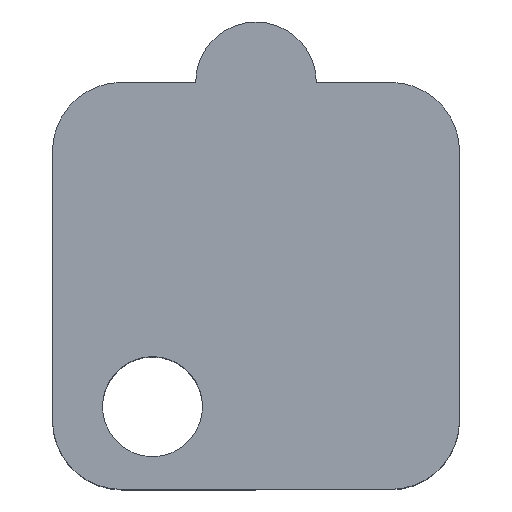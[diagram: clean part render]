
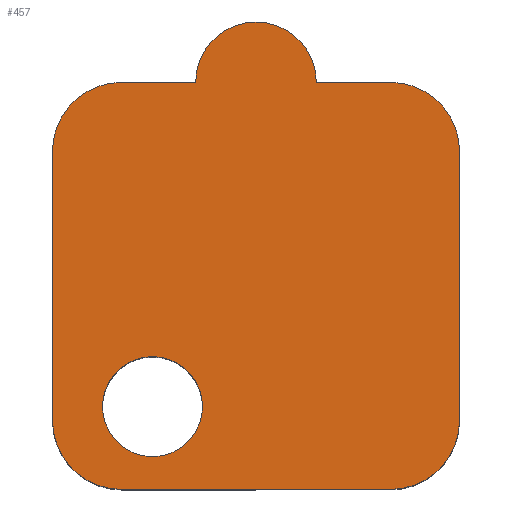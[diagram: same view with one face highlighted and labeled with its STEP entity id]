
A CAD part, top view. The second image highlights one B-rep face of the part: STEP entity #457.
In plain terms, the highlighted planar face has unit normal (0, 0, 1).
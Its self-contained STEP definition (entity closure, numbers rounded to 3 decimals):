
#73=CARTESIAN_POINT('',(-1.75,5.9,0.0));
#74=VERTEX_POINT('',#73);
#83=CARTESIAN_POINT('',(1.75,5.9,0.0));
#84=VERTEX_POINT('',#83);
#85=CARTESIAN_POINT('',(0.,5.9,0.0));
#86=DIRECTION('',(0.0,0.0,-1.0));
#87=DIRECTION('',(-1.0,0.0,0.0));
#88=AXIS2_PLACEMENT_3D('',#85,#86,#87);
#89=CIRCLE('',#88,1.75);
#90=EDGE_CURVE('',#74,#84,#89,.T.);
#133=CARTESIAN_POINT('',(3.9,5.9,0.0));
#134=VERTEX_POINT('',#133);
#135=CARTESIAN_POINT('',(1.75,5.9,0.0));
#136=DIRECTION('',(1.0,0.0,0.0));
#137=VECTOR('',#136,2.15);
#138=LINE('',#135,#137);
#139=EDGE_CURVE('',#84,#134,#138,.T.);
#157=CARTESIAN_POINT('',(-3.9,5.9,0.0));
#158=VERTEX_POINT('',#157);
#165=CARTESIAN_POINT('',(-3.9,5.9,0.0));
#166=DIRECTION('',(1.0,0.0,0.0));
#167=VECTOR('',#166,2.15);
#168=LINE('',#165,#167);
#169=EDGE_CURVE('',#158,#74,#168,.T.);
#190=CARTESIAN_POINT('',(-3.9,-5.9,0.0));
#191=VERTEX_POINT('',#190);
#198=CARTESIAN_POINT('',(-5.9,-3.9,0.0));
#199=VERTEX_POINT('',#198);
#200=CARTESIAN_POINT('',(-3.9,-3.9,0.0));
#201=DIRECTION('',(0.0,0.0,-1.0));
#202=DIRECTION('',(-0.707,-0.707,0.0));
#203=AXIS2_PLACEMENT_3D('',#200,#201,#202);
#204=CIRCLE('',#203,2.0);
#205=EDGE_CURVE('',#191,#199,#204,.T.);
#230=CARTESIAN_POINT('',(3.9,-5.9,0.0));
#231=VERTEX_POINT('',#230);
#238=CARTESIAN_POINT('',(3.9,-5.9,0.0));
#239=DIRECTION('',(-1.0,0.0,0.0));
#240=VECTOR('',#239,7.8);
#241=LINE('',#238,#240);
#242=EDGE_CURVE('',#231,#191,#241,.T.);
#314=CARTESIAN_POINT('',(5.9,-3.9,0.0));
#315=VERTEX_POINT('',#314);
#322=CARTESIAN_POINT('',(3.9,-3.9,0.0));
#323=DIRECTION('',(0.0,0.0,-1.0));
#324=DIRECTION('',(0.707,-0.707,0.0));
#325=AXIS2_PLACEMENT_3D('',#322,#323,#324);
#326=CIRCLE('',#325,2.0);
#327=EDGE_CURVE('',#315,#231,#326,.T.);
#340=CARTESIAN_POINT('',(5.9,3.9,0.0));
#341=VERTEX_POINT('',#340);
#348=CARTESIAN_POINT('',(5.9,3.9,0.0));
#349=DIRECTION('',(0.0,-1.0,0.0));
#350=VECTOR('',#349,7.8);
#351=LINE('',#348,#350);
#352=EDGE_CURVE('',#341,#315,#351,.T.);
#364=CARTESIAN_POINT('',(3.9,3.9,0.0));
#365=DIRECTION('',(0.0,0.0,-1.0));
#366=DIRECTION('',(0.707,0.707,0.0));
#367=AXIS2_PLACEMENT_3D('',#364,#365,#366);
#368=CIRCLE('',#367,2.0);
#369=EDGE_CURVE('',#134,#341,#368,.T.);
#381=CARTESIAN_POINT('',(-5.9,3.9,0.0));
#382=VERTEX_POINT('',#381);
#389=CARTESIAN_POINT('',(-3.9,3.9,0.0));
#390=DIRECTION('',(0.0,0.0,-1.0));
#391=DIRECTION('',(-0.707,0.707,0.0));
#392=AXIS2_PLACEMENT_3D('',#389,#390,#391);
#393=CIRCLE('',#392,2.0);
#394=EDGE_CURVE('',#382,#158,#393,.T.);
#408=CARTESIAN_POINT('',(-1.55,-3.5,0.0));
#409=VERTEX_POINT('',#408);
#410=CARTESIAN_POINT('',(-3.0,-3.5,0.0));
#411=DIRECTION('',(0.0,0.0,-1.0));
#412=DIRECTION('',(-1.0,0.0,0.0));
#413=AXIS2_PLACEMENT_3D('',#410,#411,#412);
#414=CIRCLE('',#413,1.45);
#415=EDGE_CURVE('',#409,#409,#414,.T.);
#426=CARTESIAN_POINT('',(-5.9,-3.9,0.0));
#427=DIRECTION('',(0.0,1.0,0.0));
#428=VECTOR('',#427,7.8);
#429=LINE('',#426,#428);
#430=EDGE_CURVE('',#199,#382,#429,.T.);
#437=CARTESIAN_POINT('',(0.,0.,0.0));
#438=DIRECTION('',(0.0,0.0,1.0));
#439=DIRECTION('',(1.0,0.0,0.0));
#440=AXIS2_PLACEMENT_3D('',#437,#438,#439);
#441=PLANE('',#440);
#442=ORIENTED_EDGE('',*,*,#169,.F.);
#443=ORIENTED_EDGE('',*,*,#394,.F.);
#444=ORIENTED_EDGE('',*,*,#430,.F.);
#445=ORIENTED_EDGE('',*,*,#205,.F.);
#446=ORIENTED_EDGE('',*,*,#242,.F.);
#447=ORIENTED_EDGE('',*,*,#327,.F.);
#448=ORIENTED_EDGE('',*,*,#352,.F.);
#449=ORIENTED_EDGE('',*,*,#369,.F.);
#450=ORIENTED_EDGE('',*,*,#139,.F.);
#451=ORIENTED_EDGE('',*,*,#90,.F.);
#452=EDGE_LOOP('',(#442,#443,#444,#445,#446,#447,#448,#449,#450,#451));
#453=FACE_OUTER_BOUND('',#452,.T.);
#454=ORIENTED_EDGE('',*,*,#415,.T.);
#455=EDGE_LOOP('',(#454));
#456=FACE_BOUND('',#455,.T.);
#457=ADVANCED_FACE('',(#453,#456),#441,.T.);
